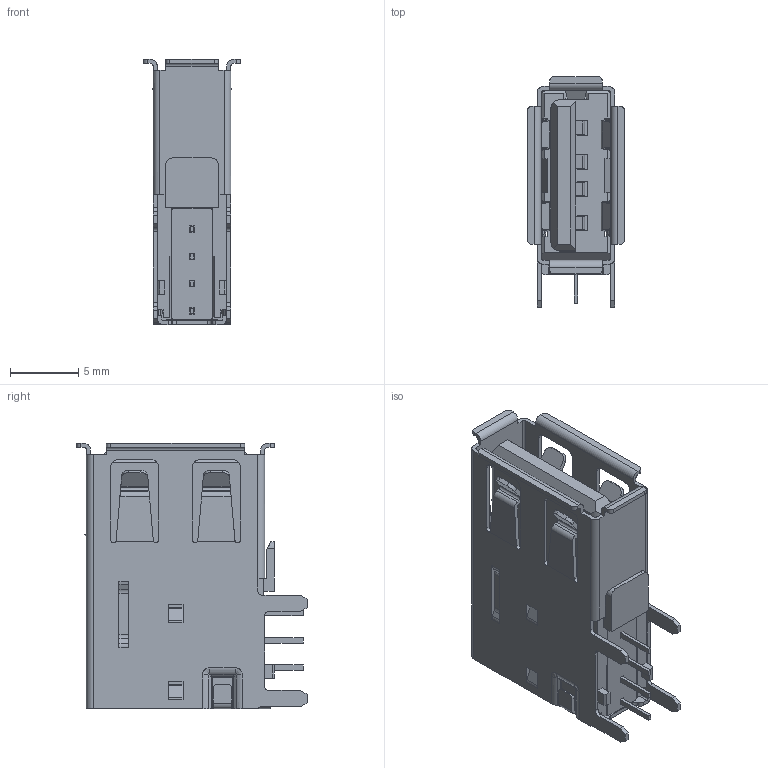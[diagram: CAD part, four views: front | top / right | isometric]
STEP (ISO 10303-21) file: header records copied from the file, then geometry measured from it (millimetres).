
FILE_DESCRIPTION (( 'STEP AP214' ), '1' );
FILE_NAME ('690C104-132-011.STEP', '2021-01-13T21:44:12', ( '' ), ( '' ), 'SwSTEP 2.0', 'SolidWorks 2020', '' );
FILE_SCHEMA (( 'AUTOMOTIVE_DESIGN' ));
Length unit declared in the file: millimetre
Products named in the file (4): 690C104-132-011; Insulator 690C104-132-011; Contacts 690C104-132-011; Shell 690C104-132-011
Assembly tree (3 placements, depth 2):
  690C104-132-011
    Insulator 690C104-132-011
    Contacts 690C104-132-011
    Shell 690C104-132-011
Bounding box: 7.12 x 16.92 x 19.5 mm (x, y, z)
Volume: 631.2 mm3; surface area: 2735.8 mm2
Topology: 6 solids, 6 shells, 1161 faces, 3332 edges, 2148 vertices
Faces by surface type: plane 797, cylinder 308, bspline 40, cone 16
Entity records: 39620 total; most frequent: CARTESIAN_POINT 9598, ORIENTED_EDGE 6664, DIRECTION 5641, EDGE_CURVE 3332, VECTOR 2573, LINE 2573, VERTEX_POINT 2148, AXIS2_PLACEMENT_3D 1534
